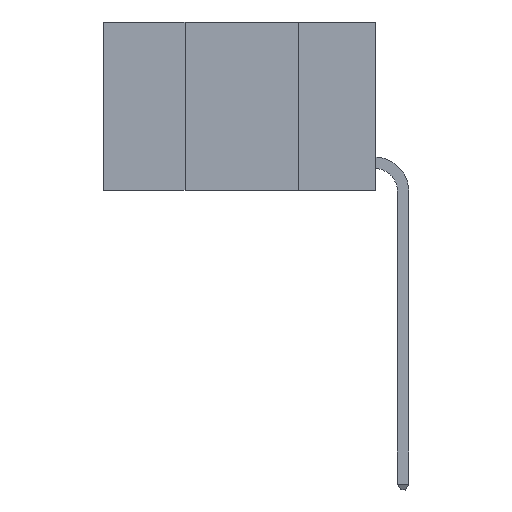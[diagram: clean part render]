
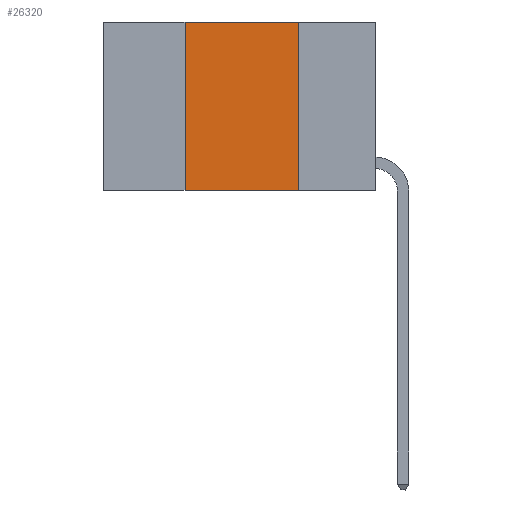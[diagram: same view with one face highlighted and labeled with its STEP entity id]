
A CAD part, left-side view. The second image highlights one B-rep face of the part: STEP entity #26320.
In plain terms, the highlighted planar face has unit normal (-1, 0, 0).
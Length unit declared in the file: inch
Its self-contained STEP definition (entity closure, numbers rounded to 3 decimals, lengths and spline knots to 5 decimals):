
#1681 = CARTESIAN_POINT ( 'NONE',  ( 0., 0.17, -0.37 ) ) ;
#2240 = VERTEX_POINT ( 'NONE', #2264 ) ;
#2264 = CARTESIAN_POINT ( 'NONE',  ( 0., 0.42, 0. ) ) ;
#2781 = CARTESIAN_POINT ( 'NONE',  ( 0., 0.42, 0. ) ) ;
#3146 = EDGE_CURVE ( 'NONE', #7073, #12438, #7228, .T. ) ;
#3613 = EDGE_CURVE ( 'NONE', #27762, #12438, #22415, .T. ) ;
#3789 = DIRECTION ( 'NONE',  ( 0., -1., 0. ) ) ;
#4762 = FACE_OUTER_BOUND ( 'NONE', #9420, .T. ) ;
#5026 = DIRECTION ( 'NONE',  ( 0., 0., 1. ) ) ;
#6038 = ORIENTED_EDGE ( 'NONE', *, *, #3613, .F. ) ;
#6450 = LINE ( 'NONE', #17234, #28527 ) ;
#7073 = VERTEX_POINT ( 'NONE', #25835 ) ;
#7213 = ORIENTED_EDGE ( 'NONE', *, *, #3146, .T. ) ;
#7228 = LINE ( 'NONE', #24829, #22788 ) ;
#9420 = EDGE_LOOP ( 'NONE', ( #6038, #23990, #9425, #7213 ) ) ;
#9425 = ORIENTED_EDGE ( 'NONE', *, *, #23790, .F. ) ;
#9617 = CARTESIAN_POINT ( 'NONE',  ( 0., 0.6, 0. ) ) ;
#10655 = CARTESIAN_POINT ( 'NONE',  ( 0., 0.17, 0. ) ) ;
#11738 = LINE ( 'NONE', #2781, #23534 ) ;
#11856 = DIRECTION ( 'NONE',  ( 0., 0., -1. ) ) ;
#12438 = VERTEX_POINT ( 'NONE', #1681 ) ;
#17234 = CARTESIAN_POINT ( 'NONE',  ( 0., 0.6, 0. ) ) ;
#19453 = DIRECTION ( 'NONE',  ( 0., -1., 0. ) ) ;
#19545 = CARTESIAN_POINT ( 'NONE',  ( 0., 0.17, 0. ) ) ;
#21721 = VECTOR ( 'NONE', #26175, 39.37008 ) ;
#22415 = LINE ( 'NONE', #19545, #21721 ) ;
#22788 = VECTOR ( 'NONE', #3789, 39.37008 ) ;
#22892 = PLANE ( 'NONE',  #24402 ) ;
#23534 = VECTOR ( 'NONE', #5026, 39.37008 ) ;
#23790 = EDGE_CURVE ( 'NONE', #7073, #2240, #11738, .T. ) ;
#23990 = ORIENTED_EDGE ( 'NONE', *, *, #25906, .F. ) ;
#24402 = AXIS2_PLACEMENT_3D ( 'NONE', #9617, #25089, #11856 ) ;
#24829 = CARTESIAN_POINT ( 'NONE',  ( 0., 0.6, -0.37 ) ) ;
#25089 = DIRECTION ( 'NONE',  ( 1., 0., 0. ) ) ;
#25835 = CARTESIAN_POINT ( 'NONE',  ( 0., 0.42, -0.37 ) ) ;
#25906 = EDGE_CURVE ( 'NONE', #2240, #27762, #6450, .T. ) ;
#26175 = DIRECTION ( 'NONE',  ( 0., 0., -1. ) ) ;
#26320 = ADVANCED_FACE ( 'NONE', ( #4762 ), #22892, .F. ) ;
#27762 = VERTEX_POINT ( 'NONE', #10655 ) ;
#28527 = VECTOR ( 'NONE', #19453, 39.37008 ) ;
